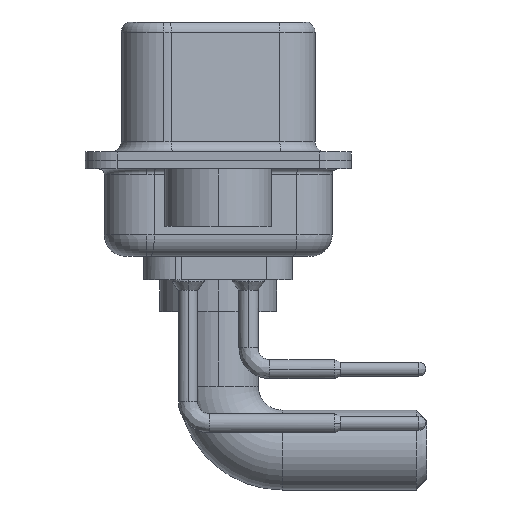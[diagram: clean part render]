
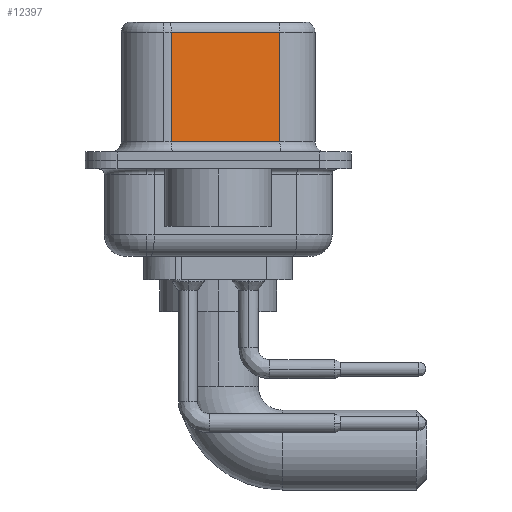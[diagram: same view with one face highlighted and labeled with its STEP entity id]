
A CAD part, left-side view. The second image highlights one B-rep face of the part: STEP entity #12397.
In plain terms, the highlighted planar face has unit normal (-0.985, -0.174, 0).
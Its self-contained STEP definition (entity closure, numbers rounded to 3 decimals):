
#157 = VECTOR ( 'NONE', #3140, 1000. ) ;
#755 = PLANE ( 'NONE',  #17363 ) ;
#3140 = DIRECTION ( 'NONE',  ( 0., 0., -1. ) ) ;
#3553 = CARTESIAN_POINT ( 'NONE',  ( 3.655, 2.203, 6.02 ) ) ;
#4075 = CARTESIAN_POINT ( 'NONE',  ( 4.555, -2.897, 0.9 ) ) ;
#4245 = CARTESIAN_POINT ( 'NONE',  ( 4.555, -2.897, 6.52 ) ) ;
#4478 = EDGE_CURVE ( 'NONE', #7628, #12875, #20047, .T. ) ;
#4632 = DIRECTION ( 'NONE',  ( 0., 0., -1. ) ) ;
#4896 = ORIENTED_EDGE ( 'NONE', *, *, #4478, .T. ) ;
#6561 = CARTESIAN_POINT ( 'NONE',  ( 3.655, 2.203, 6.52 ) ) ;
#7628 = VERTEX_POINT ( 'NONE', #3553 ) ;
#7985 = CARTESIAN_POINT ( 'NONE',  ( 3.655, 2.203, 0.9 ) ) ;
#8083 = LINE ( 'NONE', #11487, #21334 ) ;
#8275 = DIRECTION ( 'NONE',  ( -0.174, 0.985, 0. ) ) ;
#9181 = EDGE_CURVE ( 'NONE', #12875, #13328, #8083, .T. ) ;
#9971 = CARTESIAN_POINT ( 'NONE',  ( 4.555, -2.897, 6.02 ) ) ;
#11487 = CARTESIAN_POINT ( 'NONE',  ( 4.555, -2.897, 0.9 ) ) ;
#11997 = CARTESIAN_POINT ( 'NONE',  ( 4.555, -2.897, 6.52 ) ) ;
#12011 = VERTEX_POINT ( 'NONE', #18022 ) ;
#12186 = EDGE_CURVE ( 'NONE', #12011, #7628, #18593, .T. ) ;
#12397 = ADVANCED_FACE ( 'NONE', ( #16621 ), #755, .F. ) ;
#12875 = VERTEX_POINT ( 'NONE', #7985 ) ;
#13328 = VERTEX_POINT ( 'NONE', #4075 ) ;
#13447 = ORIENTED_EDGE ( 'NONE', *, *, #9181, .T. ) ;
#14741 = VECTOR ( 'NONE', #4632, 1000. ) ;
#16621 = FACE_OUTER_BOUND ( 'NONE', #17224, .T. ) ;
#17224 = EDGE_LOOP ( 'NONE', ( #19623, #19632, #4896, #13447 ) ) ;
#17363 = AXIS2_PLACEMENT_3D ( 'NONE', #4245, #21826, #18431 ) ;
#18022 = CARTESIAN_POINT ( 'NONE',  ( 4.555, -2.897, 6.02 ) ) ;
#18095 = VECTOR ( 'NONE', #8275, 1000. ) ;
#18431 = DIRECTION ( 'NONE',  ( -0.174, 0.985, 0. ) ) ;
#18593 = LINE ( 'NONE', #9971, #18095 ) ;
#18668 = LINE ( 'NONE', #11997, #157 ) ;
#18894 = EDGE_CURVE ( 'NONE', #12011, #13328, #18668, .T. ) ;
#19623 = ORIENTED_EDGE ( 'NONE', *, *, #18894, .F. ) ;
#19632 = ORIENTED_EDGE ( 'NONE', *, *, #12186, .T. ) ;
#20047 = LINE ( 'NONE', #6561, #14741 ) ;
#20214 = DIRECTION ( 'NONE',  ( 0.174, -0.985, 0. ) ) ;
#21334 = VECTOR ( 'NONE', #20214, 1000. ) ;
#21826 = DIRECTION ( 'NONE',  ( 0.985, 0.174, 0. ) ) ;
